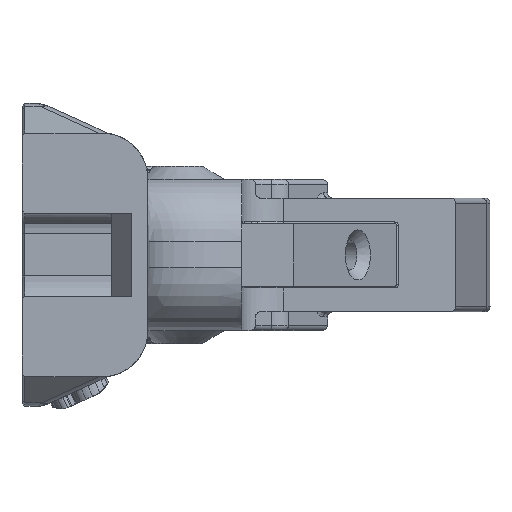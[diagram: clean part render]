
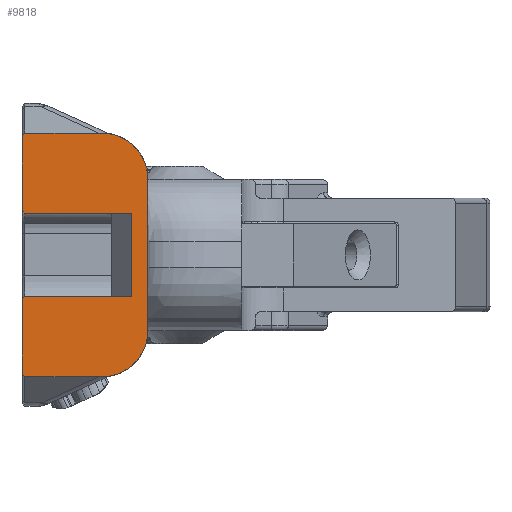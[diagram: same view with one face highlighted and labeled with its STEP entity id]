
A CAD part, left-side view. The second image highlights one B-rep face of the part: STEP entity #9818.
In plain terms, the highlighted planar face has unit normal (-1, 0, 0).
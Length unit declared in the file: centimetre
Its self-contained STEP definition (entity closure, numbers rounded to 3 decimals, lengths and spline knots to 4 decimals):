
#190=PLANE($,#10399);
#548=LINE($,#15920,#1250);
#549=LINE($,#15922,#1251);
#550=LINE($,#15924,#1252);
#551=LINE($,#15926,#1253);
#552=LINE($,#15928,#1254);
#553=LINE($,#15930,#1255);
#554=LINE($,#15933,#1256);
#555=LINE($,#15935,#1257);
#556=LINE($,#15937,#1258);
#557=LINE($,#15939,#1259);
#558=LINE($,#15941,#1260);
#559=LINE($,#15942,#1261);
#1250=VECTOR($,#11393,1.27);
#1251=VECTOR($,#11394,1.63);
#1252=VECTOR($,#11395,0.0566);
#1253=VECTOR($,#11396,1.1417);
#1254=VECTOR($,#11397,0.0566);
#1255=VECTOR($,#11398,1.172);
#1256=VECTOR($,#11401,2.3019);
#1257=VECTOR($,#11402,1.172);
#1258=VECTOR($,#11403,0.0566);
#1259=VECTOR($,#11404,1.1417);
#1260=VECTOR($,#11405,0.0566);
#1261=VECTOR($,#11406,1.63);
#2082=FACE_OUTER_BOUND($,#2679,.T.);
#2679=EDGE_LOOP($,(#6994,#6995,#6996,#6997,#6998,#6999,#7000,#7001,#7002,
#7003,#7004,#7005,#7006,#7007));
#3308=CIRCLE($,#10397,0.7057);
#3310=CIRCLE($,#10400,0.7057);
#4269=VERTEX_POINT($,#15541);
#4270=VERTEX_POINT($,#15542);
#4276=VERTEX_POINT($,#15918);
#4277=VERTEX_POINT($,#15919);
#4278=VERTEX_POINT($,#15921);
#4279=VERTEX_POINT($,#15923);
#4280=VERTEX_POINT($,#15925);
#4281=VERTEX_POINT($,#15927);
#4282=VERTEX_POINT($,#15929);
#4283=VERTEX_POINT($,#15931);
#4284=VERTEX_POINT($,#15934);
#4285=VERTEX_POINT($,#15936);
#4286=VERTEX_POINT($,#15938);
#4287=VERTEX_POINT($,#15940);
#5311=EDGE_CURVE($,#4269,#4270,#3308,.T.);
#5318=EDGE_CURVE($,#4276,#4277,#548,.F.);
#5319=EDGE_CURVE($,#4278,#4276,#549,.T.);
#5320=EDGE_CURVE($,#4279,#4278,#550,.T.);
#5321=EDGE_CURVE($,#4280,#4279,#551,.T.);
#5322=EDGE_CURVE($,#4281,#4280,#552,.T.);
#5323=EDGE_CURVE($,#4282,#4281,#553,.T.);
#5324=EDGE_CURVE($,#4283,#4282,#3310,.T.);
#5325=EDGE_CURVE($,#4270,#4283,#554,.T.);
#5326=EDGE_CURVE($,#4284,#4269,#555,.F.);
#5327=EDGE_CURVE($,#4285,#4284,#556,.T.);
#5328=EDGE_CURVE($,#4286,#4285,#557,.T.);
#5329=EDGE_CURVE($,#4287,#4286,#558,.T.);
#5330=EDGE_CURVE($,#4277,#4287,#559,.F.);
#6994=ORIENTED_EDGE($,*,*,#5318,.F.);
#6995=ORIENTED_EDGE($,*,*,#5319,.F.);
#6996=ORIENTED_EDGE($,*,*,#5320,.F.);
#6997=ORIENTED_EDGE($,*,*,#5321,.F.);
#6998=ORIENTED_EDGE($,*,*,#5322,.F.);
#6999=ORIENTED_EDGE($,*,*,#5323,.F.);
#7000=ORIENTED_EDGE($,*,*,#5324,.F.);
#7001=ORIENTED_EDGE($,*,*,#5325,.F.);
#7002=ORIENTED_EDGE($,*,*,#5311,.F.);
#7003=ORIENTED_EDGE($,*,*,#5326,.F.);
#7004=ORIENTED_EDGE($,*,*,#5327,.F.);
#7005=ORIENTED_EDGE($,*,*,#5328,.F.);
#7006=ORIENTED_EDGE($,*,*,#5329,.F.);
#7007=ORIENTED_EDGE($,*,*,#5330,.F.);
#9818=ADVANCED_FACE($,(#2082),#190,.F.);
#10397=AXIS2_PLACEMENT_3D($,#15543,#11385,#11386);
#10399=AXIS2_PLACEMENT_3D($,#15917,#11391,#11392);
#10400=AXIS2_PLACEMENT_3D($,#15932,#11399,#11400);
#11385=DIRECTION('center_axis',(1.,0.,0.));
#11386=DIRECTION('ref_axis',(0.,0.,
1.));
#11391=DIRECTION('center_axis',(1.,0.,0.));
#11392=DIRECTION('ref_axis',(0.,0.,
-1.));
#11393=DIRECTION($,(0.,0.,-1.));
#11394=DIRECTION($,(0.,-1.,0.));
#11395=DIRECTION($,(0.,-0.707,0.707));
#11396=DIRECTION($,(0.,0.,1.));
#11397=DIRECTION($,(0.,0.707,0.707));
#11398=DIRECTION($,(0.,1.,0.));
#11399=DIRECTION('center_axis',(1.,0.,0.));
#11400=DIRECTION('ref_axis',(0.,0.,
1.));
#11401=DIRECTION($,(0.,0.,-1.));
#11402=DIRECTION($,(0.,1.,0.));
#11403=DIRECTION($,(0.,-0.707,0.707));
#11404=DIRECTION($,(0.,0.,1.));
#11405=DIRECTION($,(0.,0.707,0.707));
#11406=DIRECTION($,(0.,-1.,0.));
#15541=CARTESIAN_POINT('',(-19.5982,-0.6479,1.9567));
#15542=CARTESIAN_POINT('',(-19.5982,-1.3536,1.2509));
#15543=CARTESIAN_POINT('Origin',(-19.5982,-0.6479,1.2509));
#15917=CARTESIAN_POINT('Origin',(-19.5982,-0.3095,-1.0511));
#15918=CARTESIAN_POINT('',(-19.5982,-1.1059,-0.535));
#15919=CARTESIAN_POINT('',(-19.5982,-1.1059,0.735));
#15920=CARTESIAN_POINT($,(-19.5982,-1.1059,-0.4417));
#15921=CARTESIAN_POINT('',(-19.5982,0.5241,-0.535));
#15922=CARTESIAN_POINT($,(-19.5982,1.81,-0.535));
#15923=CARTESIAN_POINT('',(-19.5982,0.5641,-0.575));
#15924=CARTESIAN_POINT($,(-19.5982,0.4547,-0.4656));
#15925=CARTESIAN_POINT('',(-19.5982,0.5641,-1.7167));
#15926=CARTESIAN_POINT($,(-19.5982,0.5641,-1.6584));
#15927=CARTESIAN_POINT('',(-19.5982,0.5241,-1.7567));
#15928=CARTESIAN_POINT($,(-19.5982,0.5021,-1.7787));
#15929=CARTESIAN_POINT('',(-19.5982,-0.6479,-1.7567));
#15930=CARTESIAN_POINT($,(-19.5982,0.1273,-1.7567));
#15931=CARTESIAN_POINT('',(-19.5982,-1.3536,-1.0509));
#15932=CARTESIAN_POINT('Origin',(-19.5982,-0.6479,-1.0509));
#15933=CARTESIAN_POINT($,(-19.5982,-1.3536,-1.051));
#15934=CARTESIAN_POINT('',(-19.5982,0.5241,1.9567));
#15935=CARTESIAN_POINT($,(-19.5982,-0.2459,1.9567));
#15936=CARTESIAN_POINT('',(-19.5982,0.5641,1.9167));
#15937=CARTESIAN_POINT($,(-19.5982,1.0776,1.4031));
#15938=CARTESIAN_POINT('',(-19.5982,0.5641,0.775));
#15939=CARTESIAN_POINT($,(-19.5982,0.5641,-1.6584));
#15940=CARTESIAN_POINT('',(-19.5982,0.5241,0.735));
#15941=CARTESIAN_POINT($,(-19.5982,-0.1209,0.0901));
#15942=CARTESIAN_POINT($,(-19.5982,1.81,0.735));
